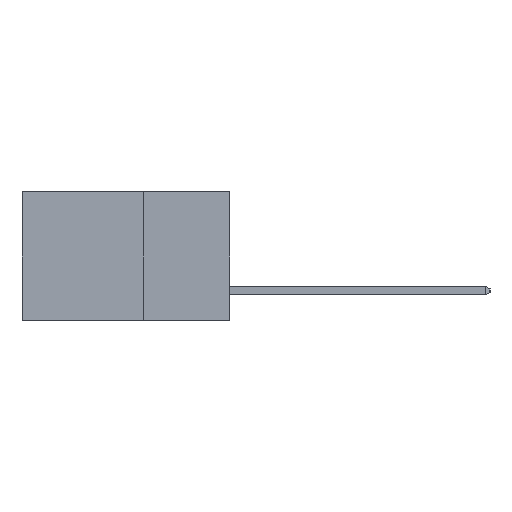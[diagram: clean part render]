
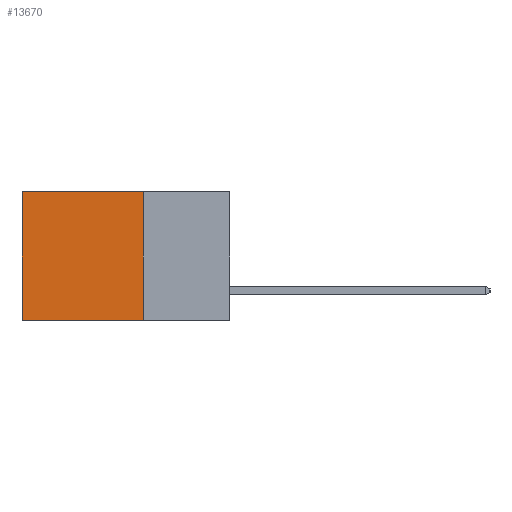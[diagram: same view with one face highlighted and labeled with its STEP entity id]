
A CAD part, left-side view. The second image highlights one B-rep face of the part: STEP entity #13670.
In plain terms, the highlighted planar face has unit normal (-1, 0, 0).
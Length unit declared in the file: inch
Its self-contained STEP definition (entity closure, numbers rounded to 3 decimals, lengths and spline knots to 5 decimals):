
#170 = ORIENTED_EDGE ( 'NONE', *, *, #3302, .T. ) ;
#302 = PLANE ( 'NONE',  #13155 ) ;
#553 = VERTEX_POINT ( 'NONE', #6747 ) ;
#997 = LINE ( 'NONE', #3893, #4480 ) ;
#1596 = DIRECTION ( 'NONE',  ( 1., 0., 0. ) ) ;
#1709 = LINE ( 'NONE', #7809, #10747 ) ;
#2857 = DIRECTION ( 'NONE',  ( 0., 1., 0. ) ) ;
#3302 = EDGE_CURVE ( 'NONE', #5982, #3718, #997, .T. ) ;
#3718 = VERTEX_POINT ( 'NONE', #8256 ) ;
#3744 = DIRECTION ( 'NONE',  ( 0., 0., -1. ) ) ;
#3768 = LINE ( 'NONE', #5088, #7077 ) ;
#3893 = CARTESIAN_POINT ( 'NONE',  ( 0.2615, 0.6, -0.37 ) ) ;
#3898 = ORIENTED_EDGE ( 'NONE', *, *, #5182, .F. ) ;
#4480 = VECTOR ( 'NONE', #3744, 39.37008 ) ;
#4610 = DIRECTION ( 'NONE',  ( 0., 1., 0. ) ) ;
#5088 = CARTESIAN_POINT ( 'NONE',  ( 0.2615, 0.25, 0. ) ) ;
#5091 = CARTESIAN_POINT ( 'NONE',  ( 0.2615, 0.25, -0.37 ) ) ;
#5182 = EDGE_CURVE ( 'NONE', #553, #8916, #10786, .T. ) ;
#5610 = CARTESIAN_POINT ( 'NONE',  ( 0.2615, 0.25, -0.37 ) ) ;
#5613 = DIRECTION ( 'NONE',  ( 0., 0., -1. ) ) ;
#5982 = VERTEX_POINT ( 'NONE', #6335 ) ;
#6288 = EDGE_CURVE ( 'NONE', #553, #5982, #3768, .T. ) ;
#6335 = CARTESIAN_POINT ( 'NONE',  ( 0.2615, 0.6, 0. ) ) ;
#6747 = CARTESIAN_POINT ( 'NONE',  ( 0.2615, 0.25, 0. ) ) ;
#7077 = VECTOR ( 'NONE', #4610, 39.37008 ) ;
#7114 = EDGE_CURVE ( 'NONE', #8916, #3718, #1709, .T. ) ;
#7809 = CARTESIAN_POINT ( 'NONE',  ( 0.2615, 0.25, -0.37 ) ) ;
#7874 = CARTESIAN_POINT ( 'NONE',  ( 0.2615, 0.25, -0.37 ) ) ;
#7938 = EDGE_LOOP ( 'NONE', ( #170, #10814, #3898, #13894 ) ) ;
#8256 = CARTESIAN_POINT ( 'NONE',  ( 0.2615, 0.6, -0.37 ) ) ;
#8916 = VERTEX_POINT ( 'NONE', #5091 ) ;
#10245 = DIRECTION ( 'NONE',  ( 0., 0., -1. ) ) ;
#10747 = VECTOR ( 'NONE', #2857, 39.37008 ) ;
#10786 = LINE ( 'NONE', #5610, #13096 ) ;
#10814 = ORIENTED_EDGE ( 'NONE', *, *, #7114, .F. ) ;
#11806 = FACE_OUTER_BOUND ( 'NONE', #7938, .T. ) ;
#13096 = VECTOR ( 'NONE', #5613, 39.37008 ) ;
#13155 = AXIS2_PLACEMENT_3D ( 'NONE', #7874, #1596, #10245 ) ;
#13670 = ADVANCED_FACE ( 'NONE', ( #11806 ), #302, .F. ) ;
#13894 = ORIENTED_EDGE ( 'NONE', *, *, #6288, .T. ) ;
